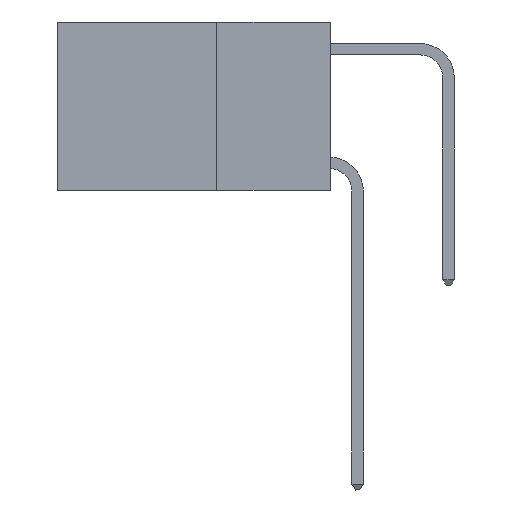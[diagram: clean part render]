
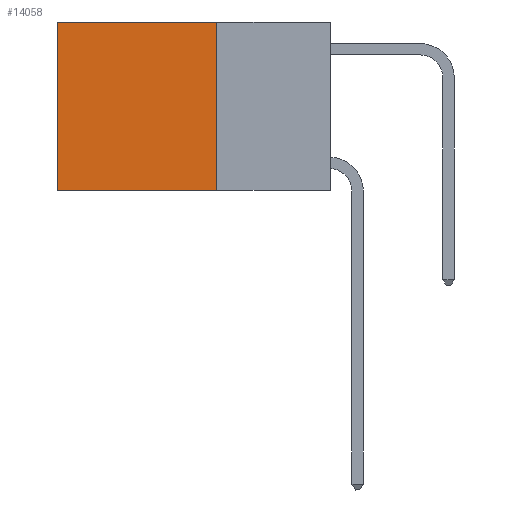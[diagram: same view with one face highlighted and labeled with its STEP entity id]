
A CAD part, left-side view. The second image highlights one B-rep face of the part: STEP entity #14058.
In plain terms, the highlighted planar face has unit normal (-1, 0, 0).
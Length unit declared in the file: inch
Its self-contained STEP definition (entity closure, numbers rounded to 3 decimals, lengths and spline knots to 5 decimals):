
#260 = DIRECTION ( 'NONE',  ( 0., 0., -1. ) ) ;
#1219 = VECTOR ( 'NONE', #20893, 39.37008 ) ;
#4130 = EDGE_CURVE ( 'NONE', #10115, #14738, #21399, .T. ) ;
#4318 = VECTOR ( 'NONE', #21461, 39.37008 ) ;
#4527 = CARTESIAN_POINT ( 'NONE',  ( 0.2625, 0.25, -0.37 ) ) ;
#5416 = LINE ( 'NONE', #28078, #30945 ) ;
#5613 = ORIENTED_EDGE ( 'NONE', *, *, #14305, .F. ) ;
#7084 = ORIENTED_EDGE ( 'NONE', *, *, #14235, .F. ) ;
#10115 = VERTEX_POINT ( 'NONE', #27490 ) ;
#10145 = EDGE_LOOP ( 'NONE', ( #18430, #7084, #5613, #25818 ) ) ;
#13296 = DIRECTION ( 'NONE',  ( 1., 0., 0. ) ) ;
#13358 = VECTOR ( 'NONE', #32754, 39.37008 ) ;
#13916 = CARTESIAN_POINT ( 'NONE',  ( 0.2625, 0.6, 0. ) ) ;
#14058 = ADVANCED_FACE ( 'NONE', ( #18304 ), #18627, .F. ) ;
#14235 = EDGE_CURVE ( 'NONE', #25219, #32410, #14281, .T. ) ;
#14281 = LINE ( 'NONE', #21626, #4318 ) ;
#14305 = EDGE_CURVE ( 'NONE', #10115, #25219, #20118, .T. ) ;
#14406 = AXIS2_PLACEMENT_3D ( 'NONE', #28960, #13296, #15461 ) ;
#14738 = VERTEX_POINT ( 'NONE', #13916 ) ;
#15263 = CARTESIAN_POINT ( 'NONE',  ( 0.2625, 0.25, 0. ) ) ;
#15461 = DIRECTION ( 'NONE',  ( 0., 0., -1. ) ) ;
#18304 = FACE_OUTER_BOUND ( 'NONE', #10145, .T. ) ;
#18430 = ORIENTED_EDGE ( 'NONE', *, *, #27388, .T. ) ;
#18627 = PLANE ( 'NONE',  #14406 ) ;
#20118 = LINE ( 'NONE', #15263, #13358 ) ;
#20893 = DIRECTION ( 'NONE',  ( 0., 1., 0. ) ) ;
#21399 = LINE ( 'NONE', #26418, #1219 ) ;
#21461 = DIRECTION ( 'NONE',  ( 0., 1., 0. ) ) ;
#21626 = CARTESIAN_POINT ( 'NONE',  ( 0.2625, 0.25, -0.37 ) ) ;
#25219 = VERTEX_POINT ( 'NONE', #4527 ) ;
#25818 = ORIENTED_EDGE ( 'NONE', *, *, #4130, .T. ) ;
#26418 = CARTESIAN_POINT ( 'NONE',  ( 0.2625, 0.25, 0. ) ) ;
#27388 = EDGE_CURVE ( 'NONE', #14738, #32410, #5416, .T. ) ;
#27490 = CARTESIAN_POINT ( 'NONE',  ( 0.2625, 0.25, 0. ) ) ;
#28078 = CARTESIAN_POINT ( 'NONE',  ( 0.2625, 0.6, 0. ) ) ;
#28960 = CARTESIAN_POINT ( 'NONE',  ( 0.2625, 0.25, 0. ) ) ;
#30945 = VECTOR ( 'NONE', #260, 39.37008 ) ;
#32410 = VERTEX_POINT ( 'NONE', #32435 ) ;
#32435 = CARTESIAN_POINT ( 'NONE',  ( 0.2625, 0.6, -0.37 ) ) ;
#32754 = DIRECTION ( 'NONE',  ( 0., 0., -1. ) ) ;
